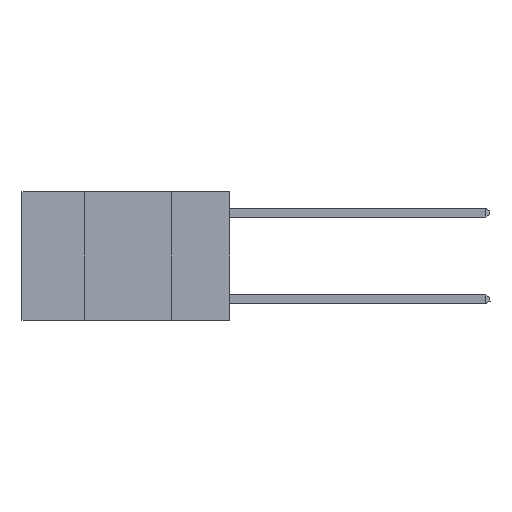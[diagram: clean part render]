
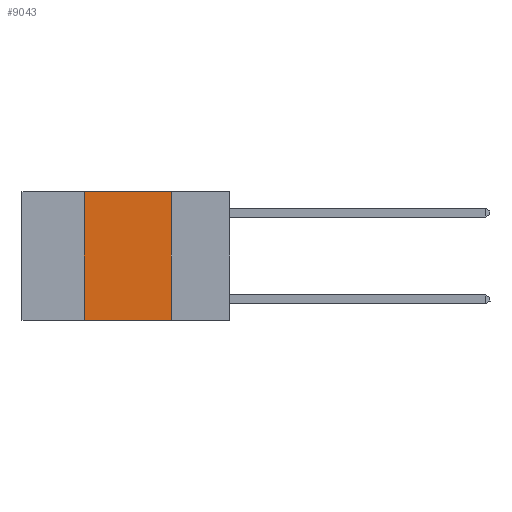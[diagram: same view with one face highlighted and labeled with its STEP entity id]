
A CAD part, left-side view. The second image highlights one B-rep face of the part: STEP entity #9043.
In plain terms, the highlighted planar face has unit normal (-1, 0, 0).
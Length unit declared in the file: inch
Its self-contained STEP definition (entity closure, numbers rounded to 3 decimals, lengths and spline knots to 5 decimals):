
#738 = ORIENTED_EDGE ( 'NONE', *, *, #5510, .F. ) ;
#1128 = EDGE_CURVE ( 'NONE', #8474, #1309, #7055, .T. ) ;
#1309 = VERTEX_POINT ( 'NONE', #3898 ) ;
#2127 = DIRECTION ( 'NONE',  ( 0., 0., 1. ) ) ;
#2363 = EDGE_LOOP ( 'NONE', ( #10903, #10914, #738, #2618 ) ) ;
#2417 = DIRECTION ( 'NONE',  ( 1., 0., 0. ) ) ;
#2618 = ORIENTED_EDGE ( 'NONE', *, *, #4690, .T. ) ;
#2646 = VERTEX_POINT ( 'NONE', #9397 ) ;
#3102 = AXIS2_PLACEMENT_3D ( 'NONE', #5253, #2417, #8685 ) ;
#3404 = CARTESIAN_POINT ( 'NONE',  ( 0., 0.42, 0. ) ) ;
#3494 = CARTESIAN_POINT ( 'NONE',  ( 0., 0.17, 0. ) ) ;
#3731 = FACE_OUTER_BOUND ( 'NONE', #2363, .T. ) ;
#3809 = DIRECTION ( 'NONE',  ( 0., -1., 0. ) ) ;
#3898 = CARTESIAN_POINT ( 'NONE',  ( 0., 0.17, 0. ) ) ;
#4499 = DIRECTION ( 'NONE',  ( 0., -1., 0. ) ) ;
#4690 = EDGE_CURVE ( 'NONE', #11074, #2646, #7334, .T. ) ;
#5253 = CARTESIAN_POINT ( 'NONE',  ( 0., 0.6, 0. ) ) ;
#5510 = EDGE_CURVE ( 'NONE', #11074, #8474, #10235, .T. ) ;
#5856 = CARTESIAN_POINT ( 'NONE',  ( 0., 0.42, 0. ) ) ;
#6090 = CARTESIAN_POINT ( 'NONE',  ( 0., 0.6, 0. ) ) ;
#7055 = LINE ( 'NONE', #6090, #8988 ) ;
#7334 = LINE ( 'NONE', #8172, #11401 ) ;
#7441 = LINE ( 'NONE', #3494, #9366 ) ;
#7873 = PLANE ( 'NONE',  #3102 ) ;
#8015 = CARTESIAN_POINT ( 'NONE',  ( 0., 0.42, -0.37 ) ) ;
#8172 = CARTESIAN_POINT ( 'NONE',  ( 0., 0.6, -0.37 ) ) ;
#8474 = VERTEX_POINT ( 'NONE', #3404 ) ;
#8685 = DIRECTION ( 'NONE',  ( 0., 0., -1. ) ) ;
#8988 = VECTOR ( 'NONE', #4499, 39.37008 ) ;
#9043 = ADVANCED_FACE ( 'NONE', ( #3731 ), #7873, .F. ) ;
#9366 = VECTOR ( 'NONE', #10353, 39.37008 ) ;
#9397 = CARTESIAN_POINT ( 'NONE',  ( 0., 0.17, -0.37 ) ) ;
#10002 = VECTOR ( 'NONE', #2127, 39.37008 ) ;
#10235 = LINE ( 'NONE', #5856, #10002 ) ;
#10353 = DIRECTION ( 'NONE',  ( 0., 0., -1. ) ) ;
#10903 = ORIENTED_EDGE ( 'NONE', *, *, #11501, .F. ) ;
#10914 = ORIENTED_EDGE ( 'NONE', *, *, #1128, .F. ) ;
#11074 = VERTEX_POINT ( 'NONE', #8015 ) ;
#11401 = VECTOR ( 'NONE', #3809, 39.37008 ) ;
#11501 = EDGE_CURVE ( 'NONE', #1309, #2646, #7441, .T. ) ;
